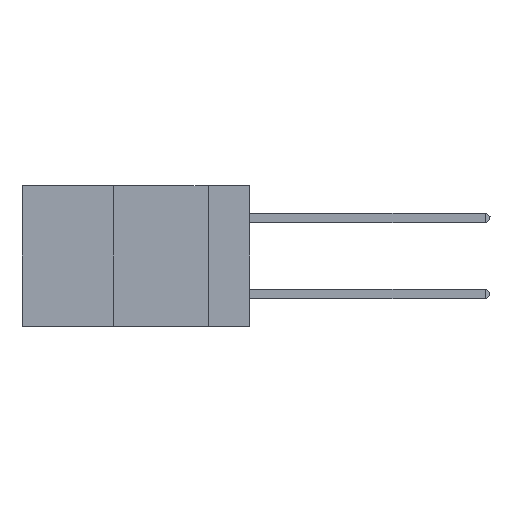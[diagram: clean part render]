
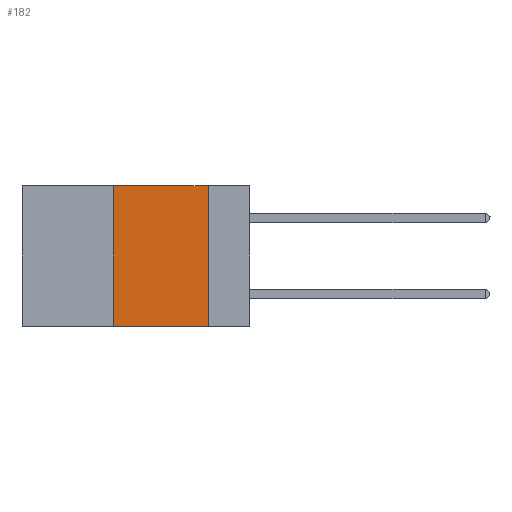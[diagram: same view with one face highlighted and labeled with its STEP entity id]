
A CAD part, left-side view. The second image highlights one B-rep face of the part: STEP entity #182.
In plain terms, the highlighted planar face has unit normal (-1, 0, 0).
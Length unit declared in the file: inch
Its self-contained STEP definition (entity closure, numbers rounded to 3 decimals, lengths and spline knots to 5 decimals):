
#128 = ORIENTED_EDGE ( 'NONE', *, *, #13317, .F. ) ;
#182 = ADVANCED_FACE ( 'NONE', ( #11255 ), #5879, .F. ) ;
#468 = DIRECTION ( 'NONE',  ( 1., 0., 0. ) ) ;
#879 = VECTOR ( 'NONE', #6329, 39.37008 ) ;
#1496 = LINE ( 'NONE', #3855, #8491 ) ;
#1544 = DIRECTION ( 'NONE',  ( 0., 0., -1. ) ) ;
#1548 = VERTEX_POINT ( 'NONE', #3049 ) ;
#2104 = CARTESIAN_POINT ( 'NONE',  ( 0., 0.6, 0. ) ) ;
#2398 = LINE ( 'NONE', #7750, #3574 ) ;
#2445 = ORIENTED_EDGE ( 'NONE', *, *, #12406, .T. ) ;
#2768 = DIRECTION ( 'NONE',  ( 0., 0., 1. ) ) ;
#3049 = CARTESIAN_POINT ( 'NONE',  ( 0., 0.11, -0.37 ) ) ;
#3150 = AXIS2_PLACEMENT_3D ( 'NONE', #6973, #468, #1544 ) ;
#3557 = EDGE_CURVE ( 'NONE', #12963, #1548, #3976, .T. ) ;
#3574 = VECTOR ( 'NONE', #6757, 39.37008 ) ;
#3792 = ORIENTED_EDGE ( 'NONE', *, *, #11695, .F. ) ;
#3855 = CARTESIAN_POINT ( 'NONE',  ( 0., 0.36, 0. ) ) ;
#3976 = LINE ( 'NONE', #8960, #8069 ) ;
#4387 = VERTEX_POINT ( 'NONE', #11979 ) ;
#5879 = PLANE ( 'NONE',  #3150 ) ;
#6329 = DIRECTION ( 'NONE',  ( 0., -1., 0. ) ) ;
#6505 = LINE ( 'NONE', #2104, #879 ) ;
#6757 = DIRECTION ( 'NONE',  ( 0., -1., 0. ) ) ;
#6973 = CARTESIAN_POINT ( 'NONE',  ( 0., 0.6, 0. ) ) ;
#7750 = CARTESIAN_POINT ( 'NONE',  ( 0., 0.6, -0.37 ) ) ;
#8069 = VECTOR ( 'NONE', #13711, 39.37008 ) ;
#8491 = VECTOR ( 'NONE', #2768, 39.37008 ) ;
#8960 = CARTESIAN_POINT ( 'NONE',  ( 0., 0.11, 0. ) ) ;
#9110 = CARTESIAN_POINT ( 'NONE',  ( 0., 0.36, 0. ) ) ;
#11255 = FACE_OUTER_BOUND ( 'NONE', #11407, .T. ) ;
#11267 = ORIENTED_EDGE ( 'NONE', *, *, #3557, .F. ) ;
#11407 = EDGE_LOOP ( 'NONE', ( #11267, #128, #3792, #2445 ) ) ;
#11695 = EDGE_CURVE ( 'NONE', #4387, #12601, #1496, .T. ) ;
#11979 = CARTESIAN_POINT ( 'NONE',  ( 0., 0.36, -0.37 ) ) ;
#12406 = EDGE_CURVE ( 'NONE', #4387, #1548, #2398, .T. ) ;
#12601 = VERTEX_POINT ( 'NONE', #9110 ) ;
#12963 = VERTEX_POINT ( 'NONE', #14164 ) ;
#13317 = EDGE_CURVE ( 'NONE', #12601, #12963, #6505, .T. ) ;
#13711 = DIRECTION ( 'NONE',  ( 0., 0., -1. ) ) ;
#14164 = CARTESIAN_POINT ( 'NONE',  ( 0., 0.11, 0. ) ) ;
